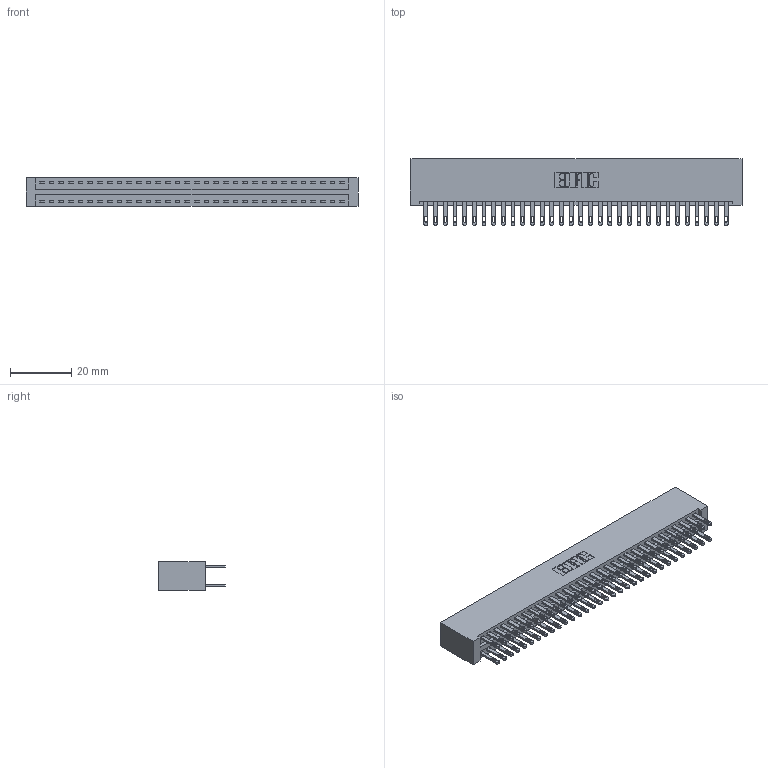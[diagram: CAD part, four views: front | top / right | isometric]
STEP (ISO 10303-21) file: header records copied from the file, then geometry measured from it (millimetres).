
FILE_DESCRIPTION (( 'STEP AP203' ), '1' );
FILE_NAME ('346-064-500-201.STEP', '2022-05-24T14:41:22', ( '' ), ( '' ), 'SwSTEP 2.0', 'SolidWorks 2020', '' );
FILE_SCHEMA (( 'CONFIG_CONTROL_DESIGN' ));
Length unit declared in the file: inch
Products named in the file (3): 346 Part_No Mounting Lugs; 345-292-001_345-293-100; 346-064-500-201
Assembly tree (65 placements, depth 2):
  346-064-500-201
    346 Part_No Mounting Lugs
    345-292-001_345-293-100  x64
Bounding box: 108.84 x 21.84 x 9.4 mm (x, y, z)
Volume: 11304.3 mm3; surface area: 16214.4 mm2
Topology: 65 solids, 65 shells, 3186 faces, 9713 edges, 6474 vertices
Faces by surface type: plane 1928, cylinder 1258
Entity records: 21883 total; most frequent: CARTESIAN_POINT 3616, ORIENTED_EDGE 3550, DIRECTION 3235, EDGE_CURVE 1775, LINE 1519, VECTOR 1519, VERTEX_POINT 1182, AXIS2_PLACEMENT_3D 858
